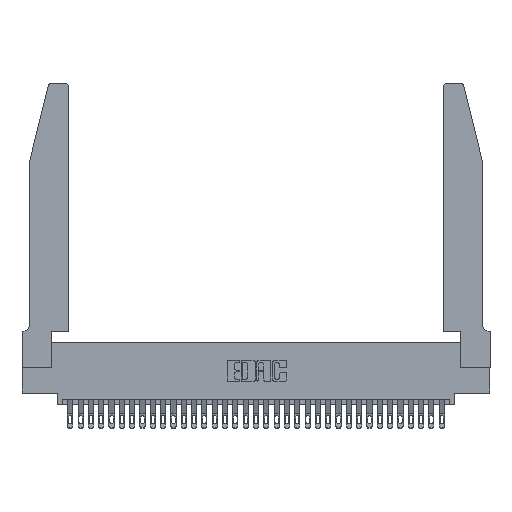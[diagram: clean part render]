
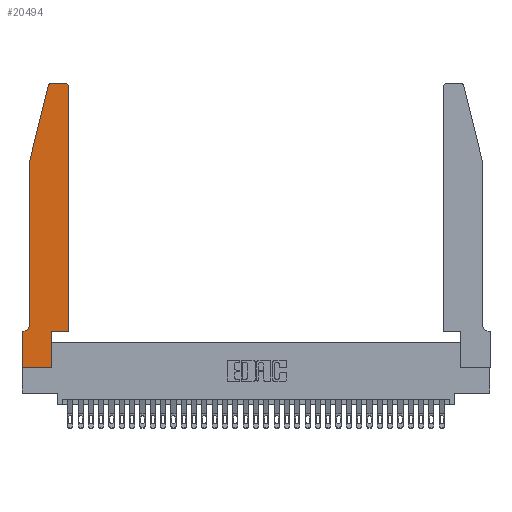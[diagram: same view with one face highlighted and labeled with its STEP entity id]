
A CAD part, top view. The second image highlights one B-rep face of the part: STEP entity #20494.
In plain terms, the highlighted planar face has unit normal (0, 0, 1).
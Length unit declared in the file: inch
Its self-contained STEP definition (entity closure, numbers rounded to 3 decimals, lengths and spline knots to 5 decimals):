
#139 = CARTESIAN_POINT ( 'NONE',  ( 0.4505, 0.35, 0.37 ) ) ;
#629 = CARTESIAN_POINT ( 'NONE',  ( 0., 0.35, 0.37 ) ) ;
#1601 = EDGE_CURVE ( 'NONE', #1768, #10138, #22678, .T. ) ;
#1685 = DIRECTION ( 'NONE',  ( -1., 0., 0. ) ) ;
#1768 = VERTEX_POINT ( 'NONE', #9780 ) ;
#1810 = CARTESIAN_POINT ( 'NONE',  ( 0.2865, 0., 0.37 ) ) ;
#2188 = FACE_OUTER_BOUND ( 'NONE', #25465, .T. ) ;
#2451 = ORIENTED_EDGE ( 'NONE', *, *, #28358, .T. ) ;
#2588 = DIRECTION ( 'NONE',  ( 1., 0., 0. ) ) ;
#2844 = ORIENTED_EDGE ( 'NONE', *, *, #26903, .T. ) ;
#4167 = CARTESIAN_POINT ( 'NONE',  ( 0.25487, 2.72718, 0.37 ) ) ;
#4637 = VECTOR ( 'NONE', #22708, 39.37008 ) ;
#4657 = LINE ( 'NONE', #34857, #10530 ) ;
#5159 = CARTESIAN_POINT ( 'NONE',  ( 0.284, 2.72, 0.37 ) ) ;
#5852 = CARTESIAN_POINT ( 'NONE',  ( 0., 0., 0.37 ) ) ;
#6336 = DIRECTION ( 'NONE',  ( -0.239, -0.971, 0. ) ) ;
#6471 = ORIENTED_EDGE ( 'NONE', *, *, #24622, .T. ) ;
#6724 = ORIENTED_EDGE ( 'NONE', *, *, #1601, .T. ) ;
#6740 = DIRECTION ( 'NONE',  ( 0., 0., -1. ) ) ;
#6818 = ORIENTED_EDGE ( 'NONE', *, *, #31307, .T. ) ;
#6989 = VECTOR ( 'NONE', #1685, 39.37008 ) ;
#7686 = AXIS2_PLACEMENT_3D ( 'NONE', #32349, #27044, #16277 ) ;
#7969 = DIRECTION ( 'NONE',  ( 1., 0., 0. ) ) ;
#8673 = CARTESIAN_POINT ( 'NONE',  ( 0.0755, 2., 0.37 ) ) ;
#8777 = AXIS2_PLACEMENT_3D ( 'NONE', #29636, #18760, #2588 ) ;
#9607 = CARTESIAN_POINT ( 'NONE',  ( 0.284, 2.75, 0.37 ) ) ;
#9780 = CARTESIAN_POINT ( 'NONE',  ( 0.0755, 0.42, 0.37 ) ) ;
#9830 = DIRECTION ( 'NONE',  ( 1., 0., 0. ) ) ;
#10138 = VERTEX_POINT ( 'NONE', #25500 ) ;
#10530 = VECTOR ( 'NONE', #18715, 39.37008 ) ;
#10593 = LINE ( 'NONE', #17959, #17749 ) ;
#10627 = EDGE_CURVE ( 'NONE', #12762, #16926, #31111, .T. ) ;
#10676 = VERTEX_POINT ( 'NONE', #629 ) ;
#10763 = ORIENTED_EDGE ( 'NONE', *, *, #34127, .T. ) ;
#11713 = ORIENTED_EDGE ( 'NONE', *, *, #15006, .T. ) ;
#11760 = LINE ( 'NONE', #27925, #4637 ) ;
#12011 = CARTESIAN_POINT ( 'NONE',  ( 0., 0., 0.37 ) ) ;
#12315 = LINE ( 'NONE', #18019, #25451 ) ;
#12726 = LINE ( 'NONE', #27801, #26315 ) ;
#12762 = VERTEX_POINT ( 'NONE', #4167 ) ;
#13966 = DIRECTION ( 'NONE',  ( 0., -1., 0. ) ) ;
#14180 = VERTEX_POINT ( 'NONE', #12011 ) ;
#14263 = EDGE_CURVE ( 'NONE', #28613, #29778, #10593, .T. ) ;
#14288 = EDGE_CURVE ( 'NONE', #29495, #28613, #26666, .T. ) ;
#15006 = EDGE_CURVE ( 'NONE', #23033, #12762, #30823, .T. ) ;
#15129 = ORIENTED_EDGE ( 'NONE', *, *, #14288, .T. ) ;
#15767 = CARTESIAN_POINT ( 'NONE',  ( 0.4505, 2.72, 0.37 ) ) ;
#16277 = DIRECTION ( 'NONE',  ( 1., 0., 0. ) ) ;
#16483 = DIRECTION ( 'NONE',  ( 1., 0., 0. ) ) ;
#16603 = VERTEX_POINT ( 'NONE', #19595 ) ;
#16668 = ORIENTED_EDGE ( 'NONE', *, *, #32280, .T. ) ;
#16926 = VERTEX_POINT ( 'NONE', #28398 ) ;
#17610 = DIRECTION ( 'NONE',  ( -1., 0., 0. ) ) ;
#17749 = VECTOR ( 'NONE', #28603, 39.37008 ) ;
#17959 = CARTESIAN_POINT ( 'NONE',  ( 0.4505, 0.35, 0.37 ) ) ;
#18019 = CARTESIAN_POINT ( 'NONE',  ( 0., 0., 0.37 ) ) ;
#18715 = DIRECTION ( 'NONE',  ( -1., 0., 0. ) ) ;
#18760 = DIRECTION ( 'NONE',  ( 0., 0., 1. ) ) ;
#19595 = CARTESIAN_POINT ( 'NONE',  ( 0.4205, 2.75, 0.37 ) ) ;
#19748 = VERTEX_POINT ( 'NONE', #1810 ) ;
#20494 = ADVANCED_FACE ( 'NONE', ( #2188 ), #32681, .T. ) ;
#20528 = AXIS2_PLACEMENT_3D ( 'NONE', #5159, #29380, #7969 ) ;
#20797 = ORIENTED_EDGE ( 'NONE', *, *, #14263, .T. ) ;
#21574 = VECTOR ( 'NONE', #16483, 39.37008 ) ;
#22678 = CIRCLE ( 'NONE', #25212, 0.07 ) ;
#22708 = DIRECTION ( 'NONE',  ( 0., 1., 0. ) ) ;
#23033 = VERTEX_POINT ( 'NONE', #9607 ) ;
#24622 = EDGE_CURVE ( 'NONE', #29778, #16603, #26561, .T. ) ;
#24982 = DIRECTION ( 'NONE',  ( 0., -1., 0. ) ) ;
#25212 = AXIS2_PLACEMENT_3D ( 'NONE', #27998, #6740, #17610 ) ;
#25451 = VECTOR ( 'NONE', #9830, 39.37008 ) ;
#25465 = EDGE_LOOP ( 'NONE', ( #31905, #11713, #30816, #6818, #6724, #2844, #10763, #2451, #16668, #15129, #20797, #6471 ) ) ;
#25500 = CARTESIAN_POINT ( 'NONE',  ( 0.0055, 0.35, 0.37 ) ) ;
#26076 = VECTOR ( 'NONE', #13966, 39.37008 ) ;
#26315 = VECTOR ( 'NONE', #24982, 39.37008 ) ;
#26561 = CIRCLE ( 'NONE', #8777, 0.03 ) ;
#26666 = LINE ( 'NONE', #26707, #21574 ) ;
#26707 = CARTESIAN_POINT ( 'NONE',  ( 0.4505, 0.35, 0.37 ) ) ;
#26903 = EDGE_CURVE ( 'NONE', #10138, #10676, #28553, .T. ) ;
#27044 = DIRECTION ( 'NONE',  ( 0., 0., 1. ) ) ;
#27801 = CARTESIAN_POINT ( 'NONE',  ( 0.0755, 2., 0.37 ) ) ;
#27925 = CARTESIAN_POINT ( 'NONE',  ( 0.2865, 0.35, 0.37 ) ) ;
#27998 = CARTESIAN_POINT ( 'NONE',  ( 0.0055, 0.42, 0.37 ) ) ;
#28358 = EDGE_CURVE ( 'NONE', #14180, #19748, #12315, .T. ) ;
#28398 = CARTESIAN_POINT ( 'NONE',  ( 0.0755, 2., 0.37 ) ) ;
#28553 = LINE ( 'NONE', #31090, #6989 ) ;
#28603 = DIRECTION ( 'NONE',  ( 0., 1., 0. ) ) ;
#28613 = VERTEX_POINT ( 'NONE', #139 ) ;
#29380 = DIRECTION ( 'NONE',  ( 0., 0., 1. ) ) ;
#29495 = VERTEX_POINT ( 'NONE', #30418 ) ;
#29636 = CARTESIAN_POINT ( 'NONE',  ( 0.4205, 2.72, 0.37 ) ) ;
#29778 = VERTEX_POINT ( 'NONE', #15767 ) ;
#29842 = EDGE_CURVE ( 'NONE', #16603, #23033, #4657, .T. ) ;
#30418 = CARTESIAN_POINT ( 'NONE',  ( 0.2865, 0.35, 0.37 ) ) ;
#30816 = ORIENTED_EDGE ( 'NONE', *, *, #10627, .T. ) ;
#30823 = CIRCLE ( 'NONE', #20528, 0.03 ) ;
#31090 = CARTESIAN_POINT ( 'NONE',  ( 0.0755, 0.35, 0.37 ) ) ;
#31111 = LINE ( 'NONE', #8673, #32784 ) ;
#31307 = EDGE_CURVE ( 'NONE', #16926, #1768, #12726, .T. ) ;
#31905 = ORIENTED_EDGE ( 'NONE', *, *, #29842, .T. ) ;
#32280 = EDGE_CURVE ( 'NONE', #19748, #29495, #11760, .T. ) ;
#32349 = CARTESIAN_POINT ( 'NONE',  ( 0., 0.35, 0.37 ) ) ;
#32681 = PLANE ( 'NONE',  #7686 ) ;
#32784 = VECTOR ( 'NONE', #6336, 39.37008 ) ;
#34127 = EDGE_CURVE ( 'NONE', #10676, #14180, #34515, .T. ) ;
#34515 = LINE ( 'NONE', #5852, #26076 ) ;
#34857 = CARTESIAN_POINT ( 'NONE',  ( 0.2605, 2.75, 0.37 ) ) ;
